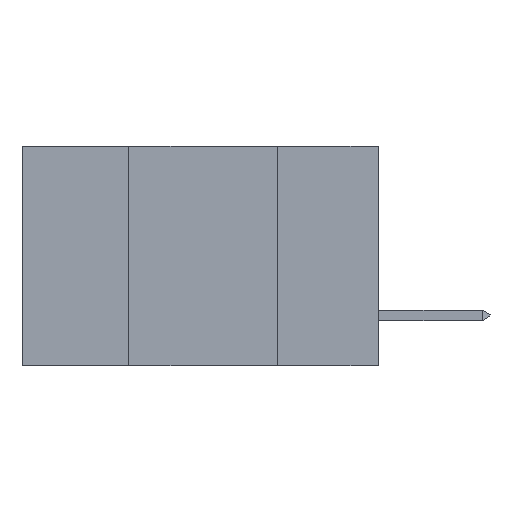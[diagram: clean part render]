
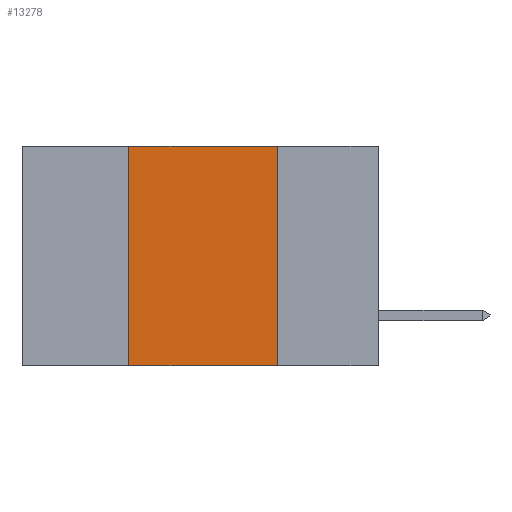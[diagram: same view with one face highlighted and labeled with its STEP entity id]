
A CAD part, left-side view. The second image highlights one B-rep face of the part: STEP entity #13278.
In plain terms, the highlighted planar face has unit normal (-1, 0, 0).
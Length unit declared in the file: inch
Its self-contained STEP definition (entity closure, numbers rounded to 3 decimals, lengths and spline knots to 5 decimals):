
#621 = EDGE_CURVE ( 'NONE', #11270, #2082, #5749, .T. ) ;
#890 = CARTESIAN_POINT ( 'NONE',  ( 0., 0.42, 0. ) ) ;
#915 = ORIENTED_EDGE ( 'NONE', *, *, #621, .F. ) ;
#1103 = LINE ( 'NONE', #4879, #9346 ) ;
#1460 = CARTESIAN_POINT ( 'NONE',  ( 0., 0.17, -0.37 ) ) ;
#1996 = EDGE_CURVE ( 'NONE', #2082, #2395, #3177, .T. ) ;
#2010 = CARTESIAN_POINT ( 'NONE',  ( 0., 0.6, 0. ) ) ;
#2082 = VERTEX_POINT ( 'NONE', #5525 ) ;
#2395 = VERTEX_POINT ( 'NONE', #12634 ) ;
#3008 = DIRECTION ( 'NONE',  ( 1., 0., 0. ) ) ;
#3037 = DIRECTION ( 'NONE',  ( 0., -1., 0. ) ) ;
#3177 = LINE ( 'NONE', #2010, #12812 ) ;
#3243 = CARTESIAN_POINT ( 'NONE',  ( 0., 0.42, -0.37 ) ) ;
#4879 = CARTESIAN_POINT ( 'NONE',  ( 0., 0.6, -0.37 ) ) ;
#5525 = CARTESIAN_POINT ( 'NONE',  ( 0., 0.42, 0. ) ) ;
#5749 = LINE ( 'NONE', #890, #7649 ) ;
#6390 = PLANE ( 'NONE',  #14129 ) ;
#6474 = DIRECTION ( 'NONE',  ( 0., 0., 1. ) ) ;
#6599 = ORIENTED_EDGE ( 'NONE', *, *, #11064, .F. ) ;
#6871 = EDGE_CURVE ( 'NONE', #11270, #9713, #1103, .T. ) ;
#7536 = DIRECTION ( 'NONE',  ( 0., 0., -1. ) ) ;
#7649 = VECTOR ( 'NONE', #6474, 39.37008 ) ;
#9108 = LINE ( 'NONE', #10649, #10155 ) ;
#9346 = VECTOR ( 'NONE', #9564, 39.37008 ) ;
#9564 = DIRECTION ( 'NONE',  ( 0., -1., 0. ) ) ;
#9713 = VERTEX_POINT ( 'NONE', #1460 ) ;
#10155 = VECTOR ( 'NONE', #13830, 39.37008 ) ;
#10649 = CARTESIAN_POINT ( 'NONE',  ( 0., 0.17, 0. ) ) ;
#11064 = EDGE_CURVE ( 'NONE', #2395, #9713, #9108, .T. ) ;
#11270 = VERTEX_POINT ( 'NONE', #3243 ) ;
#11445 = ORIENTED_EDGE ( 'NONE', *, *, #1996, .F. ) ;
#12634 = CARTESIAN_POINT ( 'NONE',  ( 0., 0.17, 0. ) ) ;
#12812 = VECTOR ( 'NONE', #3037, 39.37008 ) ;
#12861 = FACE_OUTER_BOUND ( 'NONE', #13527, .T. ) ;
#13278 = ADVANCED_FACE ( 'NONE', ( #12861 ), #6390, .F. ) ;
#13527 = EDGE_LOOP ( 'NONE', ( #6599, #11445, #915, #14058 ) ) ;
#13830 = DIRECTION ( 'NONE',  ( 0., 0., -1. ) ) ;
#14058 = ORIENTED_EDGE ( 'NONE', *, *, #6871, .T. ) ;
#14061 = CARTESIAN_POINT ( 'NONE',  ( 0., 0.6, 0. ) ) ;
#14129 = AXIS2_PLACEMENT_3D ( 'NONE', #14061, #3008, #7536 ) ;
